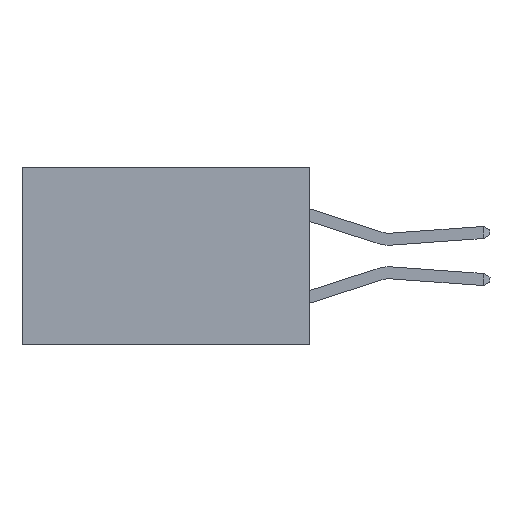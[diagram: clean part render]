
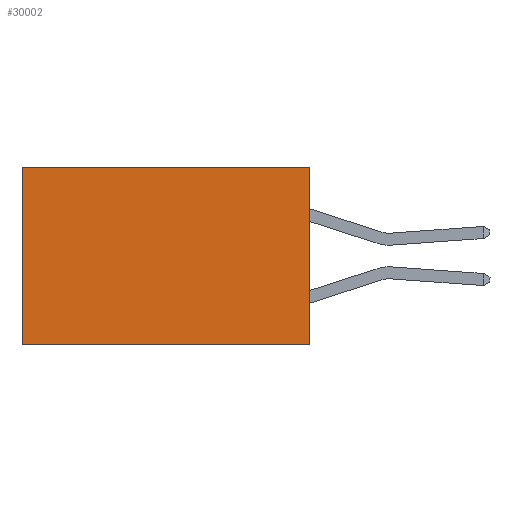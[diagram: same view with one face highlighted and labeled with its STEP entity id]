
A CAD part, left-side view. The second image highlights one B-rep face of the part: STEP entity #30002.
In plain terms, the highlighted planar face has unit normal (-1, 0, 0).
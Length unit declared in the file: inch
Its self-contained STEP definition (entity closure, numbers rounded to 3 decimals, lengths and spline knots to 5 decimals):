
#859 = CARTESIAN_POINT ( 'NONE',  ( 0.298, 0.6, 0. ) ) ;
#994 = ORIENTED_EDGE ( 'NONE', *, *, #13446, .F. ) ;
#1727 = CARTESIAN_POINT ( 'NONE',  ( 0.298, 0., 0. ) ) ;
#3668 = LINE ( 'NONE', #25456, #15747 ) ;
#3876 = VERTEX_POINT ( 'NONE', #859 ) ;
#4401 = AXIS2_PLACEMENT_3D ( 'NONE', #13596, #13705, #30433 ) ;
#6064 = EDGE_CURVE ( 'NONE', #23537, #9044, #3668, .T. ) ;
#6184 = CARTESIAN_POINT ( 'NONE',  ( 0.298, 0.6, -0.37 ) ) ;
#6525 = VECTOR ( 'NONE', #23494, 39.37008 ) ;
#7911 = LINE ( 'NONE', #10323, #23297 ) ;
#9044 = VERTEX_POINT ( 'NONE', #6184 ) ;
#9969 = LINE ( 'NONE', #21023, #22062 ) ;
#10205 = EDGE_LOOP ( 'NONE', ( #20955, #29474, #994, #12415 ) ) ;
#10323 = CARTESIAN_POINT ( 'NONE',  ( 0.298, 0., 0. ) ) ;
#11030 = EDGE_CURVE ( 'NONE', #15722, #3876, #25015, .T. ) ;
#11279 = PLANE ( 'NONE',  #4401 ) ;
#12415 = ORIENTED_EDGE ( 'NONE', *, *, #11030, .T. ) ;
#13446 = EDGE_CURVE ( 'NONE', #15722, #23537, #7911, .T. ) ;
#13596 = CARTESIAN_POINT ( 'NONE',  ( 0.298, 0., 0. ) ) ;
#13705 = DIRECTION ( 'NONE',  ( 1., 0., 0. ) ) ;
#13828 = DIRECTION ( 'NONE',  ( 0., 0., -1. ) ) ;
#15062 = EDGE_CURVE ( 'NONE', #3876, #9044, #9969, .T. ) ;
#15722 = VERTEX_POINT ( 'NONE', #30826 ) ;
#15747 = VECTOR ( 'NONE', #30158, 39.37008 ) ;
#20021 = DIRECTION ( 'NONE',  ( 0., 0., -1. ) ) ;
#20955 = ORIENTED_EDGE ( 'NONE', *, *, #15062, .T. ) ;
#21023 = CARTESIAN_POINT ( 'NONE',  ( 0.298, 0.6, 0. ) ) ;
#22062 = VECTOR ( 'NONE', #13828, 39.37008 ) ;
#23297 = VECTOR ( 'NONE', #20021, 39.37008 ) ;
#23494 = DIRECTION ( 'NONE',  ( 0., 1., 0. ) ) ;
#23537 = VERTEX_POINT ( 'NONE', #30497 ) ;
#25015 = LINE ( 'NONE', #1727, #6525 ) ;
#25456 = CARTESIAN_POINT ( 'NONE',  ( 0.298, 0., -0.37 ) ) ;
#28576 = FACE_OUTER_BOUND ( 'NONE', #10205, .T. ) ;
#29474 = ORIENTED_EDGE ( 'NONE', *, *, #6064, .F. ) ;
#30002 = ADVANCED_FACE ( 'NONE', ( #28576 ), #11279, .F. ) ;
#30158 = DIRECTION ( 'NONE',  ( 0., 1., 0. ) ) ;
#30433 = DIRECTION ( 'NONE',  ( 0., 0., -1. ) ) ;
#30497 = CARTESIAN_POINT ( 'NONE',  ( 0.298, 0., -0.37 ) ) ;
#30826 = CARTESIAN_POINT ( 'NONE',  ( 0.298, 0., 0. ) ) ;
